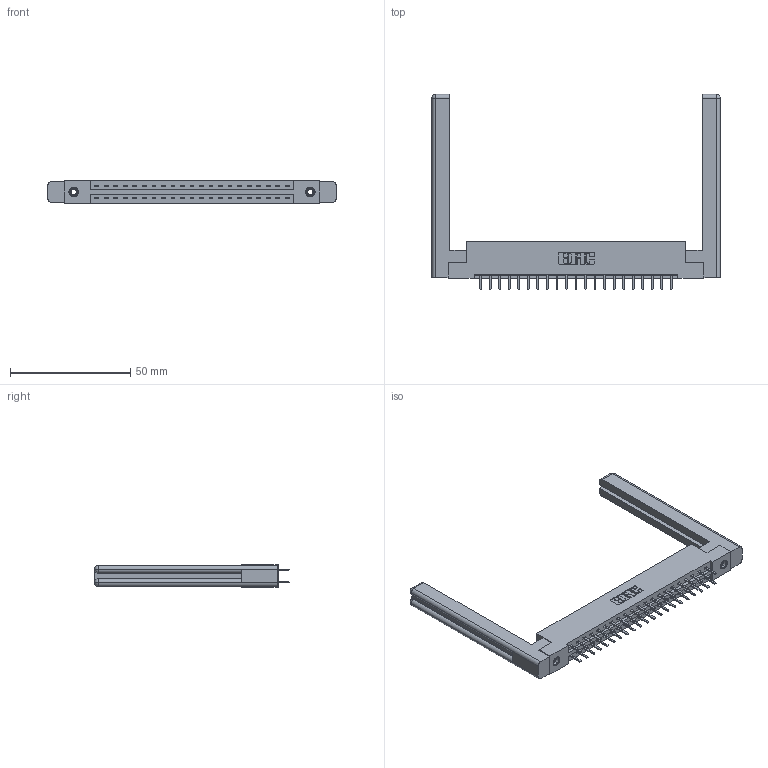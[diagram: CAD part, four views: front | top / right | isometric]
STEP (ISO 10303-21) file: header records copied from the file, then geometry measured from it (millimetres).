
FILE_DESCRIPTION (( 'STEP AP203' ), '1' );
FILE_NAME ('337-042-520-258.STEP', '2019-10-09T12:02:30', ( '' ), ( '' ), 'SwSTEP 2.0', 'SolidWorks 2016', '' );
FILE_SCHEMA (( 'CONFIG_CONTROL_DESIGN' ));
Length unit declared in the file: inch
Products named in the file (5): 345-292-001_345-293-120; 307-220-058; 337-042-520-258; 337 Part_Flush Mounting Lugs - 0.156 Dia-TI; 345-250-001_345-250-001-102
Assembly tree (47 placements, depth 2):
  337-042-520-258
    337 Part_Flush Mounting Lugs - 0.156 Dia-TI
    345-292-001_345-293-120  x42
    345-250-001_345-250-001-102  x2
    307-220-058  x2
Bounding box: 119.84 x 81.11 x 9.4 mm (x, y, z)
Volume: 19473.7 mm3; surface area: 18730.8 mm2
Topology: 47 solids, 47 shells, 2692 faces, 7763 edges, 5050 vertices
Faces by surface type: plane 1834, cylinder 834, cone 12, torus 12
Entity records: 21746 total; most frequent: CARTESIAN_POINT 3701, ORIENTED_EDGE 3564, DIRECTION 3190, EDGE_CURVE 1782, LINE 1602, VECTOR 1602, VERTEX_POINT 1178, AXIS2_PLACEMENT_3D 794
